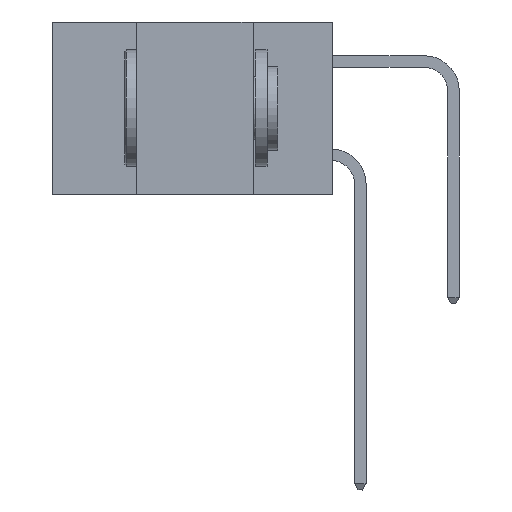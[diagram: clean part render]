
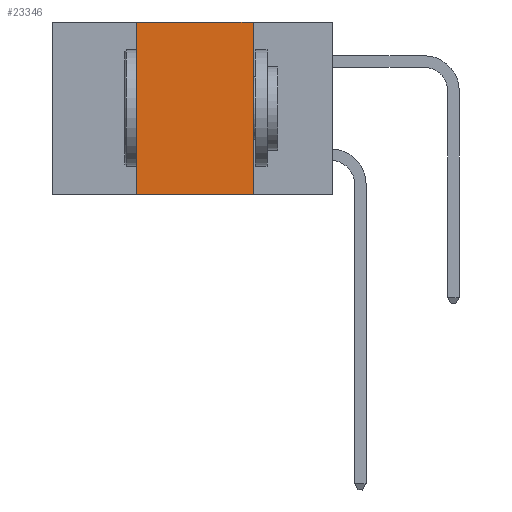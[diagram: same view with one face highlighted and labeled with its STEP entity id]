
A CAD part, left-side view. The second image highlights one B-rep face of the part: STEP entity #23346.
In plain terms, the highlighted planar face has unit normal (-1, 0, 0).
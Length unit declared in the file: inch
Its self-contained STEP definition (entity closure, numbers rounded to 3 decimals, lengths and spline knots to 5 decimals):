
#282 = CARTESIAN_POINT ( 'NONE',  ( 0., 0.6, -0.37 ) ) ;
#459 = DIRECTION ( 'NONE',  ( 0., -1., 0. ) ) ;
#867 = PLANE ( 'NONE',  #10248 ) ;
#1724 = CARTESIAN_POINT ( 'NONE',  ( 0., 0.42, -0.37 ) ) ;
#2113 = ORIENTED_EDGE ( 'NONE', *, *, #12339, .F. ) ;
#2448 = EDGE_CURVE ( 'NONE', #15807, #8833, #4405, .T. ) ;
#3753 = DIRECTION ( 'NONE',  ( 0., 0., -1. ) ) ;
#4405 = LINE ( 'NONE', #24573, #7537 ) ;
#4641 = EDGE_CURVE ( 'NONE', #20004, #15807, #10001, .T. ) ;
#4801 = ORIENTED_EDGE ( 'NONE', *, *, #22935, .T. ) ;
#6397 = ORIENTED_EDGE ( 'NONE', *, *, #4641, .F. ) ;
#6590 = LINE ( 'NONE', #282, #24565 ) ;
#7015 = VERTEX_POINT ( 'NONE', #16175 ) ;
#7537 = VECTOR ( 'NONE', #459, 39.37008 ) ;
#8833 = VERTEX_POINT ( 'NONE', #15884 ) ;
#10001 = LINE ( 'NONE', #1724, #11963 ) ;
#10248 = AXIS2_PLACEMENT_3D ( 'NONE', #18383, #20637, #22613 ) ;
#11865 = DIRECTION ( 'NONE',  ( 0., 0., 1. ) ) ;
#11926 = CARTESIAN_POINT ( 'NONE',  ( 0., 0.17, -0.37 ) ) ;
#11963 = VECTOR ( 'NONE', #11865, 39.37008 ) ;
#12339 = EDGE_CURVE ( 'NONE', #8833, #7015, #16011, .T. ) ;
#14501 = DIRECTION ( 'NONE',  ( 0., -1., 0. ) ) ;
#14862 = ORIENTED_EDGE ( 'NONE', *, *, #2448, .F. ) ;
#15035 = VECTOR ( 'NONE', #3753, 39.37008 ) ;
#15509 = EDGE_LOOP ( 'NONE', ( #2113, #14862, #6397, #4801 ) ) ;
#15807 = VERTEX_POINT ( 'NONE', #19071 ) ;
#15884 = CARTESIAN_POINT ( 'NONE',  ( 0., 0.17, 0. ) ) ;
#16011 = LINE ( 'NONE', #11926, #15035 ) ;
#16175 = CARTESIAN_POINT ( 'NONE',  ( 0., 0.17, -0.37 ) ) ;
#18383 = CARTESIAN_POINT ( 'NONE',  ( 0., 0.6, 0. ) ) ;
#19071 = CARTESIAN_POINT ( 'NONE',  ( 0., 0.42, 0. ) ) ;
#20004 = VERTEX_POINT ( 'NONE', #24357 ) ;
#20637 = DIRECTION ( 'NONE',  ( 1., 0., 0. ) ) ;
#20896 = FACE_OUTER_BOUND ( 'NONE', #15509, .T. ) ;
#22613 = DIRECTION ( 'NONE',  ( 0., 0., -1. ) ) ;
#22935 = EDGE_CURVE ( 'NONE', #20004, #7015, #6590, .T. ) ;
#23346 = ADVANCED_FACE ( 'NONE', ( #20896 ), #867, .F. ) ;
#24357 = CARTESIAN_POINT ( 'NONE',  ( 0., 0.42, -0.37 ) ) ;
#24565 = VECTOR ( 'NONE', #14501, 39.37008 ) ;
#24573 = CARTESIAN_POINT ( 'NONE',  ( 0., 0.6, 0. ) ) ;
